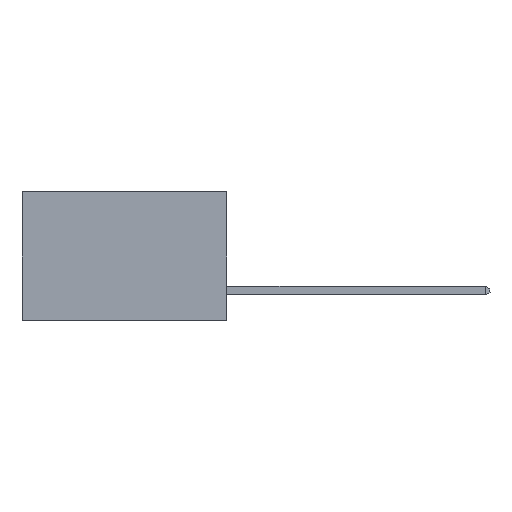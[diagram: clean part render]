
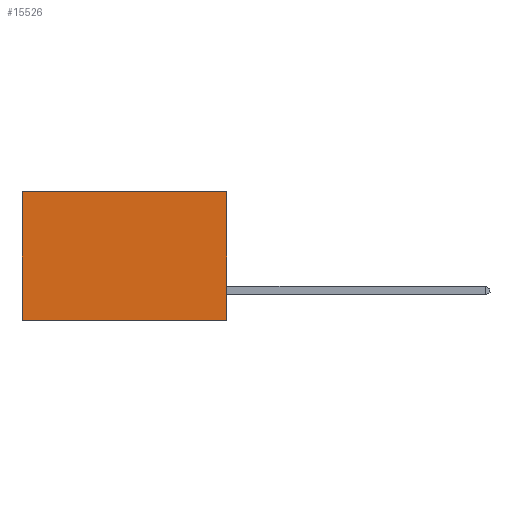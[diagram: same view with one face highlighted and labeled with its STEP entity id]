
A CAD part, left-side view. The second image highlights one B-rep face of the part: STEP entity #15526.
In plain terms, the highlighted planar face has unit normal (-1, 0, 0).
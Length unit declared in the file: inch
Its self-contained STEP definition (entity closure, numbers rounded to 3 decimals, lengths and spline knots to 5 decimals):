
#387 = CARTESIAN_POINT ( 'NONE',  ( 0.277, 0.59, -0.37 ) ) ;
#866 = VERTEX_POINT ( 'NONE', #387 ) ;
#945 = VERTEX_POINT ( 'NONE', #1697 ) ;
#1697 = CARTESIAN_POINT ( 'NONE',  ( 0.277, 0.59, 0. ) ) ;
#2924 = DIRECTION ( 'NONE',  ( 0., 0., -1. ) ) ;
#4258 = VERTEX_POINT ( 'NONE', #11254 ) ;
#4440 = ORIENTED_EDGE ( 'NONE', *, *, #11949, .T. ) ;
#5154 = LINE ( 'NONE', #15538, #11739 ) ;
#5545 = CARTESIAN_POINT ( 'NONE',  ( 0.277, 0., -0.37 ) ) ;
#5638 = CARTESIAN_POINT ( 'NONE',  ( 0.277, 0.59, -0.37 ) ) ;
#5779 = CARTESIAN_POINT ( 'NONE',  ( 0.277, 0., -0.37 ) ) ;
#5950 = VECTOR ( 'NONE', #14837, 39.37008 ) ;
#6497 = DIRECTION ( 'NONE',  ( 0., 0., -1. ) ) ;
#6797 = CARTESIAN_POINT ( 'NONE',  ( 0.277, 0., -0.37 ) ) ;
#6839 = PLANE ( 'NONE',  #16313 ) ;
#7871 = EDGE_CURVE ( 'NONE', #4258, #945, #13754, .T. ) ;
#8164 = DIRECTION ( 'NONE',  ( 0., 0., -1. ) ) ;
#9931 = VECTOR ( 'NONE', #13995, 39.37008 ) ;
#10130 = CARTESIAN_POINT ( 'NONE',  ( 0.277, 0., 0. ) ) ;
#10525 = VERTEX_POINT ( 'NONE', #6797 ) ;
#11254 = CARTESIAN_POINT ( 'NONE',  ( 0.277, 0., 0. ) ) ;
#11561 = LINE ( 'NONE', #5638, #14912 ) ;
#11739 = VECTOR ( 'NONE', #6497, 39.37008 ) ;
#11949 = EDGE_CURVE ( 'NONE', #945, #866, #11561, .T. ) ;
#12517 = LINE ( 'NONE', #5779, #5950 ) ;
#12944 = EDGE_CURVE ( 'NONE', #4258, #10525, #5154, .T. ) ;
#13059 = ORIENTED_EDGE ( 'NONE', *, *, #13698, .F. ) ;
#13461 = ORIENTED_EDGE ( 'NONE', *, *, #12944, .F. ) ;
#13698 = EDGE_CURVE ( 'NONE', #10525, #866, #12517, .T. ) ;
#13754 = LINE ( 'NONE', #10130, #9931 ) ;
#13995 = DIRECTION ( 'NONE',  ( 0., 1., 0. ) ) ;
#14410 = FACE_OUTER_BOUND ( 'NONE', #16044, .T. ) ;
#14837 = DIRECTION ( 'NONE',  ( 0., 1., 0. ) ) ;
#14912 = VECTOR ( 'NONE', #2924, 39.37008 ) ;
#15526 = ADVANCED_FACE ( 'NONE', ( #14410 ), #6839, .F. ) ;
#15538 = CARTESIAN_POINT ( 'NONE',  ( 0.277, 0., -0.37 ) ) ;
#15855 = DIRECTION ( 'NONE',  ( 1., 0., 0. ) ) ;
#16044 = EDGE_LOOP ( 'NONE', ( #4440, #13059, #13461, #16736 ) ) ;
#16313 = AXIS2_PLACEMENT_3D ( 'NONE', #5545, #15855, #8164 ) ;
#16736 = ORIENTED_EDGE ( 'NONE', *, *, #7871, .T. ) ;
